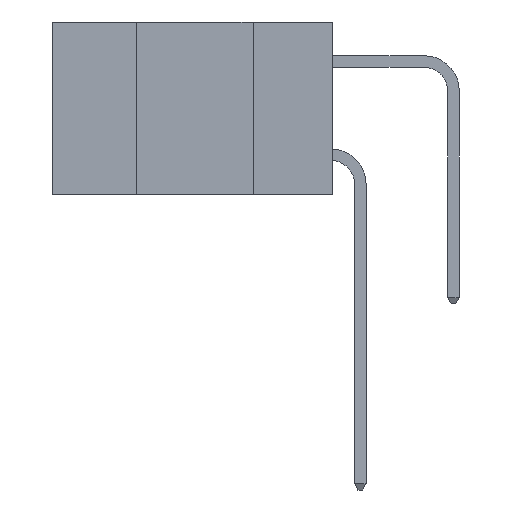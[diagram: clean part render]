
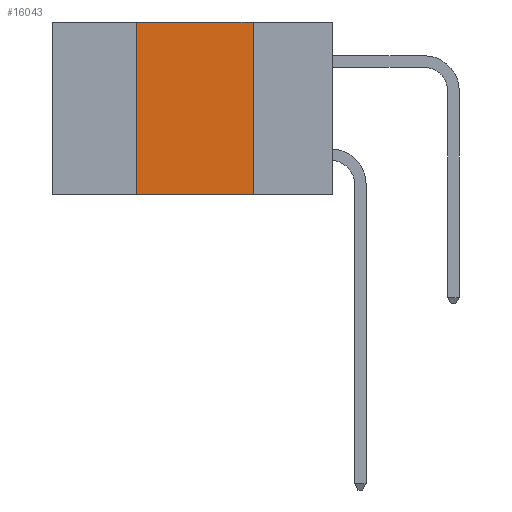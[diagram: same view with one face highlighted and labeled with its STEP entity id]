
A CAD part, left-side view. The second image highlights one B-rep face of the part: STEP entity #16043.
In plain terms, the highlighted planar face has unit normal (-1, 0, 0).
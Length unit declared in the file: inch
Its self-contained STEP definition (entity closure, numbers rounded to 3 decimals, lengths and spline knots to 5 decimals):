
#13 = FACE_OUTER_BOUND ( 'NONE', #469, .T. ) ;
#26 = CARTESIAN_POINT ( 'NONE',  ( 0., 0.17, 0. ) ) ;
#100 = EDGE_CURVE ( 'NONE', #8390, #8998, #13418, .T. ) ;
#469 = EDGE_LOOP ( 'NONE', ( #5695, #14726, #4551, #19467 ) ) ;
#1481 = DIRECTION ( 'NONE',  ( 1., 0., 0. ) ) ;
#3791 = VECTOR ( 'NONE', #17255, 39.37008 ) ;
#4060 = DIRECTION ( 'NONE',  ( 0., -1., 0. ) ) ;
#4551 = ORIENTED_EDGE ( 'NONE', *, *, #18889, .F. ) ;
#4859 = LINE ( 'NONE', #18976, #8481 ) ;
#5695 = ORIENTED_EDGE ( 'NONE', *, *, #6457, .F. ) ;
#6317 = VERTEX_POINT ( 'NONE', #18942 ) ;
#6457 = EDGE_CURVE ( 'NONE', #8998, #6317, #16837, .T. ) ;
#6724 = VECTOR ( 'NONE', #16876, 39.37008 ) ;
#8390 = VERTEX_POINT ( 'NONE', #18678 ) ;
#8481 = VECTOR ( 'NONE', #11609, 39.37008 ) ;
#8998 = VERTEX_POINT ( 'NONE', #26 ) ;
#9351 = VECTOR ( 'NONE', #4060, 39.37008 ) ;
#9533 = CARTESIAN_POINT ( 'NONE',  ( 0., 0.6, 0. ) ) ;
#10685 = PLANE ( 'NONE',  #12029 ) ;
#11609 = DIRECTION ( 'NONE',  ( 0., -1., 0. ) ) ;
#11738 = CARTESIAN_POINT ( 'NONE',  ( 0., 0.42, -0.37 ) ) ;
#12029 = AXIS2_PLACEMENT_3D ( 'NONE', #18101, #1481, #12200 ) ;
#12200 = DIRECTION ( 'NONE',  ( 0., 0., -1. ) ) ;
#13418 = LINE ( 'NONE', #9533, #9351 ) ;
#14726 = ORIENTED_EDGE ( 'NONE', *, *, #100, .F. ) ;
#16043 = ADVANCED_FACE ( 'NONE', ( #13 ), #10685, .F. ) ;
#16837 = LINE ( 'NONE', #17259, #3791 ) ;
#16876 = DIRECTION ( 'NONE',  ( 0., 0., 1. ) ) ;
#17255 = DIRECTION ( 'NONE',  ( 0., 0., -1. ) ) ;
#17259 = CARTESIAN_POINT ( 'NONE',  ( 0., 0.17, -0.37 ) ) ;
#17938 = EDGE_CURVE ( 'NONE', #18468, #6317, #4859, .T. ) ;
#18101 = CARTESIAN_POINT ( 'NONE',  ( 0., 0.6, 0. ) ) ;
#18259 = LINE ( 'NONE', #18325, #6724 ) ;
#18325 = CARTESIAN_POINT ( 'NONE',  ( 0., 0.42, -0.37 ) ) ;
#18468 = VERTEX_POINT ( 'NONE', #11738 ) ;
#18678 = CARTESIAN_POINT ( 'NONE',  ( 0., 0.42, 0. ) ) ;
#18889 = EDGE_CURVE ( 'NONE', #18468, #8390, #18259, .T. ) ;
#18942 = CARTESIAN_POINT ( 'NONE',  ( 0., 0.17, -0.37 ) ) ;
#18976 = CARTESIAN_POINT ( 'NONE',  ( 0., 0.6, -0.37 ) ) ;
#19467 = ORIENTED_EDGE ( 'NONE', *, *, #17938, .T. ) ;
